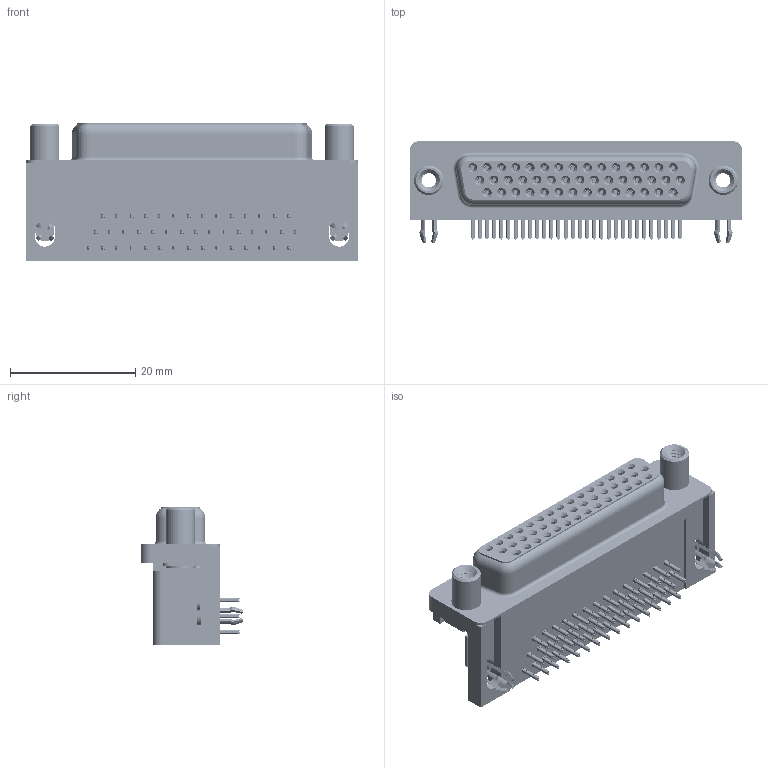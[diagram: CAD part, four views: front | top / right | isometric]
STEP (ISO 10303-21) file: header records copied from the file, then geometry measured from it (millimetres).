
FILE_DESCRIPTION (( 'STEP AP203' ), '1' );
FILE_NAME ('634-044-263-540.STEP', '2018-11-10T00:32:02', ( '' ), ( '' ), 'SwSTEP 2.0', 'SolidWorks 2016', '' );
FILE_SCHEMA (( 'CONFIG_CONTROL_DESIGN' ));
Length unit declared in the file: millimetre
Products named in the file (8): 634 Shell_44 Socket; Contact Bottom; Contact Middle; Contact Top; 4 Prong Board Lock; Round Threaded Standoff; 634-044-263-540; 634 Housing_44 Socket
Assembly tree (50 placements, depth 2):
  634-044-263-540
    634 Housing_44 Socket
    634 Shell_44 Socket
    Contact Bottom  x14
    Contact Middle  x15
    Contact Top  x15
    4 Prong Board Lock  x2
    Round Threaded Standoff  x2
Bounding box: 53.04 x 16.25 x 22.1 mm (x, y, z)
Volume: 9456.4 mm3; surface area: 13552.9 mm2
Topology: 50 solids, 50 shells, 6651 faces, 17542 edges, 11026 vertices
Faces by surface type: plane 2963, bspline 1544, cylinder 1510, cone 580, torus 54
Entity records: 46933 total; most frequent: CARTESIAN_POINT 14098, ORIENTED_EDGE 6540, DIRECTION 6020, EDGE_CURVE 3270, VECTOR 2164, LINE 2164, VERTEX_POINT 2096, AXIS2_PLACEMENT_3D 1928
